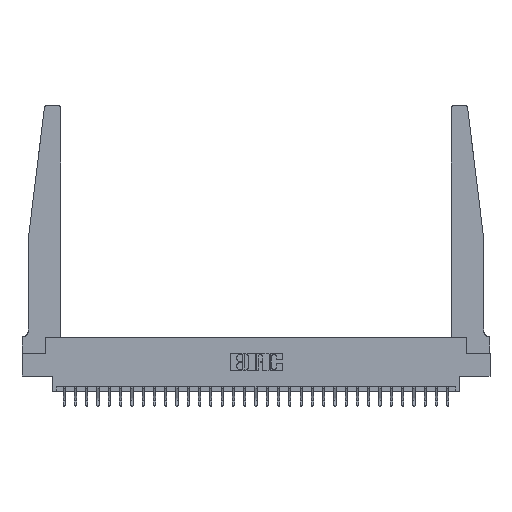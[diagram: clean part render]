
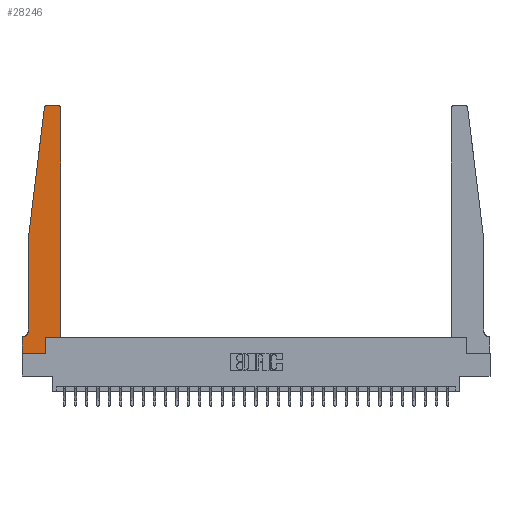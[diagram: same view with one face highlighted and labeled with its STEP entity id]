
A CAD part, top view. The second image highlights one B-rep face of the part: STEP entity #28246.
In plain terms, the highlighted planar face has unit normal (0, 0, 1).
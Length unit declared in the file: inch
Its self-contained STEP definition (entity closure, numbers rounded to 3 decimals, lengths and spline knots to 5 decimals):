
#41 = VECTOR ( 'NONE', #8136, 39.37008 ) ;
#341 = DIRECTION ( 'NONE',  ( 1., 0., 0. ) ) ;
#466 = CIRCLE ( 'NONE', #17093, 0.03 ) ;
#663 = FACE_OUTER_BOUND ( 'NONE', #11536, .T. ) ;
#838 = LINE ( 'NONE', #7801, #13449 ) ;
#1031 = ORIENTED_EDGE ( 'NONE', *, *, #2581, .T. ) ;
#1100 = CARTESIAN_POINT ( 'NONE',  ( 0., 0.1875, 0.37 ) ) ;
#1261 = DIRECTION ( 'NONE',  ( 0., 1., 0. ) ) ;
#1475 = DIRECTION ( 'NONE',  ( 1., 0., 0. ) ) ;
#1795 = VECTOR ( 'NONE', #1261, 39.37008 ) ;
#2581 = EDGE_CURVE ( 'NONE', #13372, #25763, #5997, .T. ) ;
#2959 = DIRECTION ( 'NONE',  ( 0., -1., 0. ) ) ;
#3012 = CARTESIAN_POINT ( 'NONE',  ( 0.065, 0.2375, 0.37 ) ) ;
#3028 = PLANE ( 'NONE',  #3092 ) ;
#3055 = CARTESIAN_POINT ( 'NONE',  ( 0.395, 2.72, 0.37 ) ) ;
#3092 = AXIS2_PLACEMENT_3D ( 'NONE', #1100, #16593, #23253 ) ;
#3280 = AXIS2_PLACEMENT_3D ( 'NONE', #10961, #13181, #23243 ) ;
#3397 = CARTESIAN_POINT ( 'NONE',  ( 0., 0., 0.37 ) ) ;
#3946 = CARTESIAN_POINT ( 'NONE',  ( 0.25, 2.75, 0.37 ) ) ;
#4197 = CARTESIAN_POINT ( 'NONE',  ( 0.2605, 0.18, 0.37 ) ) ;
#4422 = CARTESIAN_POINT ( 'NONE',  ( 0.065, 1.25, 0.37 ) ) ;
#4691 = ORIENTED_EDGE ( 'NONE', *, *, #26102, .T. ) ;
#4986 = DIRECTION ( 'NONE',  ( 1., 0., 0. ) ) ;
#5133 = DIRECTION ( 'NONE',  ( 0., 1., 0. ) ) ;
#5612 = LINE ( 'NONE', #21534, #8575 ) ;
#5997 = LINE ( 'NONE', #19691, #21953 ) ;
#6355 = CARTESIAN_POINT ( 'NONE',  ( 0.24675, 2.72367, 0.37 ) ) ;
#6360 = CARTESIAN_POINT ( 'NONE',  ( 0.395, 2.75, 0.37 ) ) ;
#6679 = CARTESIAN_POINT ( 'NONE',  ( 0.425, 0.18, 0.37 ) ) ;
#6717 = VECTOR ( 'NONE', #20669, 39.37008 ) ;
#7073 = ORIENTED_EDGE ( 'NONE', *, *, #19573, .T. ) ;
#7225 = VERTEX_POINT ( 'NONE', #17032 ) ;
#7440 = ORIENTED_EDGE ( 'NONE', *, *, #13970, .T. ) ;
#7603 = VERTEX_POINT ( 'NONE', #25593 ) ;
#7801 = CARTESIAN_POINT ( 'NONE',  ( 0.425, 0.18, 0.37 ) ) ;
#8092 = VECTOR ( 'NONE', #24959, 39.37008 ) ;
#8136 = DIRECTION ( 'NONE',  ( -1., 0., 0. ) ) ;
#8575 = VECTOR ( 'NONE', #2959, 39.37008 ) ;
#8946 = DIRECTION ( 'NONE',  ( 0., 0., 1. ) ) ;
#9116 = VECTOR ( 'NONE', #1475, 39.37008 ) ;
#9205 = CARTESIAN_POINT ( 'NONE',  ( 0.065, 1.25, 0.37 ) ) ;
#9310 = DIRECTION ( 'NONE',  ( 0., 0., 1. ) ) ;
#10724 = VERTEX_POINT ( 'NONE', #4422 ) ;
#10961 = CARTESIAN_POINT ( 'NONE',  ( 0.015, 0.2375, 0.37 ) ) ;
#10976 = ORIENTED_EDGE ( 'NONE', *, *, #13872, .T. ) ;
#11051 = CARTESIAN_POINT ( 'NONE',  ( 0.2605, 0.18, 0.37 ) ) ;
#11372 = CARTESIAN_POINT ( 'NONE',  ( 0.015, 0.1875, 0.37 ) ) ;
#11536 = EDGE_LOOP ( 'NONE', ( #24392, #15392, #19593, #7440, #20707, #1031, #28589, #21865, #27057, #10976, #4691, #7073 ) ) ;
#11696 = EDGE_CURVE ( 'NONE', #18968, #13372, #18012, .T. ) ;
#12478 = VECTOR ( 'NONE', #22521, 39.37008 ) ;
#13084 = AXIS2_PLACEMENT_3D ( 'NONE', #20711, #8946, #341 ) ;
#13181 = DIRECTION ( 'NONE',  ( 0., 0., -1. ) ) ;
#13372 = VERTEX_POINT ( 'NONE', #11372 ) ;
#13449 = VECTOR ( 'NONE', #5133, 39.37008 ) ;
#13469 = CARTESIAN_POINT ( 'NONE',  ( 0., 0., 0.37 ) ) ;
#13872 = EDGE_CURVE ( 'NONE', #15709, #20780, #18149, .T. ) ;
#13970 = EDGE_CURVE ( 'NONE', #10724, #18968, #5612, .T. ) ;
#14195 = EDGE_CURVE ( 'NONE', #25382, #27935, #24203, .T. ) ;
#15392 = ORIENTED_EDGE ( 'NONE', *, *, #28407, .T. ) ;
#15524 = LINE ( 'NONE', #4197, #1795 ) ;
#15706 = LINE ( 'NONE', #13469, #12478 ) ;
#15709 = VERTEX_POINT ( 'NONE', #11051 ) ;
#15820 = CARTESIAN_POINT ( 'NONE',  ( 0.2605, 0., 0.37 ) ) ;
#16593 = DIRECTION ( 'NONE',  ( 0., 0., 1. ) ) ;
#17032 = CARTESIAN_POINT ( 'NONE',  ( 0., 0., 0.37 ) ) ;
#17093 = AXIS2_PLACEMENT_3D ( 'NONE', #3055, #9310, #4986 ) ;
#17512 = EDGE_CURVE ( 'NONE', #17545, #15709, #15524, .T. ) ;
#17545 = VERTEX_POINT ( 'NONE', #15820 ) ;
#17697 = LINE ( 'NONE', #3397, #9116 ) ;
#17866 = CIRCLE ( 'NONE', #13084, 0.03 ) ;
#18012 = CIRCLE ( 'NONE', #3280, 0.05 ) ;
#18149 = LINE ( 'NONE', #27195, #8092 ) ;
#18968 = VERTEX_POINT ( 'NONE', #3012 ) ;
#19573 = EDGE_CURVE ( 'NONE', #7603, #25382, #466, .T. ) ;
#19593 = ORIENTED_EDGE ( 'NONE', *, *, #22369, .T. ) ;
#19691 = CARTESIAN_POINT ( 'NONE',  ( 0.065, 0.1875, 0.37 ) ) ;
#20669 = DIRECTION ( 'NONE',  ( -0.122, -0.992, 0. ) ) ;
#20707 = ORIENTED_EDGE ( 'NONE', *, *, #11696, .T. ) ;
#20711 = CARTESIAN_POINT ( 'NONE',  ( 0.27653, 2.72, 0.37 ) ) ;
#20780 = VERTEX_POINT ( 'NONE', #6679 ) ;
#21534 = CARTESIAN_POINT ( 'NONE',  ( 0.065, 1.25, 0.37 ) ) ;
#21865 = ORIENTED_EDGE ( 'NONE', *, *, #24165, .T. ) ;
#21953 = VECTOR ( 'NONE', #23849, 39.37008 ) ;
#22369 = EDGE_CURVE ( 'NONE', #24197, #10724, #22732, .T. ) ;
#22521 = DIRECTION ( 'NONE',  ( 0., -1., 0. ) ) ;
#22732 = LINE ( 'NONE', #9205, #6717 ) ;
#23243 = DIRECTION ( 'NONE',  ( -1., 0., 0. ) ) ;
#23253 = DIRECTION ( 'NONE',  ( 1., 0., 0. ) ) ;
#23849 = DIRECTION ( 'NONE',  ( -1., 0., 0. ) ) ;
#24165 = EDGE_CURVE ( 'NONE', #7225, #17545, #17697, .T. ) ;
#24197 = VERTEX_POINT ( 'NONE', #6355 ) ;
#24203 = LINE ( 'NONE', #3946, #41 ) ;
#24392 = ORIENTED_EDGE ( 'NONE', *, *, #14195, .T. ) ;
#24703 = EDGE_CURVE ( 'NONE', #25763, #7225, #15706, .T. ) ;
#24959 = DIRECTION ( 'NONE',  ( 1., 0., 0. ) ) ;
#25382 = VERTEX_POINT ( 'NONE', #6360 ) ;
#25593 = CARTESIAN_POINT ( 'NONE',  ( 0.425, 2.72, 0.37 ) ) ;
#25763 = VERTEX_POINT ( 'NONE', #26116 ) ;
#26102 = EDGE_CURVE ( 'NONE', #20780, #7603, #838, .T. ) ;
#26116 = CARTESIAN_POINT ( 'NONE',  ( 0., 0.1875, 0.37 ) ) ;
#26679 = CARTESIAN_POINT ( 'NONE',  ( 0.27653, 2.75, 0.37 ) ) ;
#27057 = ORIENTED_EDGE ( 'NONE', *, *, #17512, .T. ) ;
#27195 = CARTESIAN_POINT ( 'NONE',  ( 0.425, 0.18, 0.37 ) ) ;
#27935 = VERTEX_POINT ( 'NONE', #26679 ) ;
#28246 = ADVANCED_FACE ( 'NONE', ( #663 ), #3028, .T. ) ;
#28407 = EDGE_CURVE ( 'NONE', #27935, #24197, #17866, .T. ) ;
#28589 = ORIENTED_EDGE ( 'NONE', *, *, #24703, .T. ) ;
